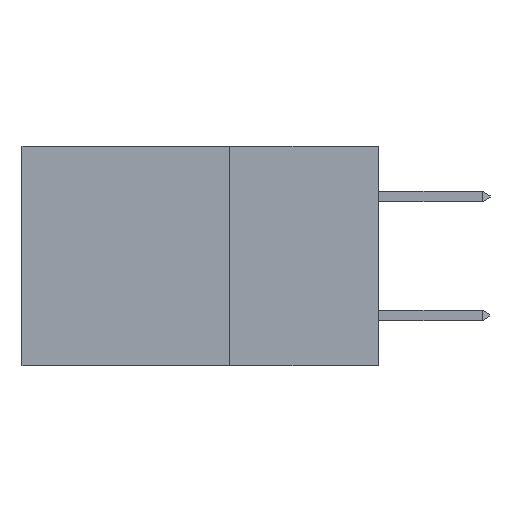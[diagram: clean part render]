
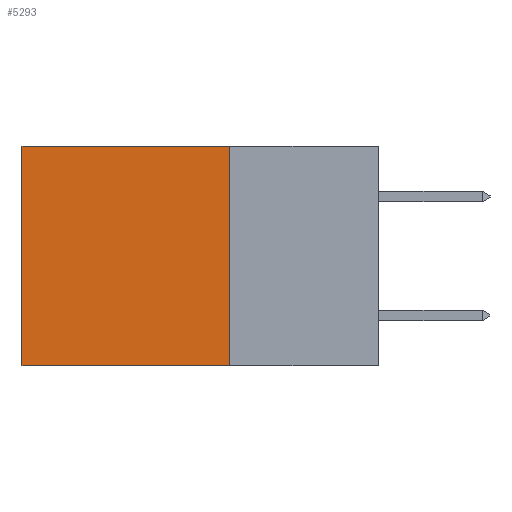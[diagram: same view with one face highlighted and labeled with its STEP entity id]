
A CAD part, left-side view. The second image highlights one B-rep face of the part: STEP entity #5293.
In plain terms, the highlighted planar face has unit normal (-1, 0, 0).
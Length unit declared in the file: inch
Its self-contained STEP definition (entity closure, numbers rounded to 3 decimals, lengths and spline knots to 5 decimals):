
#200 = VERTEX_POINT ( 'NONE', #7161 ) ;
#597 = LINE ( 'NONE', #3033, #8702 ) ;
#736 = EDGE_CURVE ( 'NONE', #4060, #6956, #4952, .T. ) ;
#774 = EDGE_CURVE ( 'NONE', #200, #6956, #8485, .T. ) ;
#1307 = EDGE_LOOP ( 'NONE', ( #2714, #2326, #4616, #5127 ) ) ;
#1610 = EDGE_CURVE ( 'NONE', #3892, #4060, #4056, .T. ) ;
#2326 = ORIENTED_EDGE ( 'NONE', *, *, #736, .F. ) ;
#2632 = CARTESIAN_POINT ( 'NONE',  ( 0.298, 0.6, -0.37 ) ) ;
#2685 = DIRECTION ( 'NONE',  ( 0., 0., -1. ) ) ;
#2714 = ORIENTED_EDGE ( 'NONE', *, *, #774, .T. ) ;
#3033 = CARTESIAN_POINT ( 'NONE',  ( 0.298, 0.25, 0. ) ) ;
#3379 = CARTESIAN_POINT ( 'NONE',  ( 0.298, 0.25, -0.37 ) ) ;
#3395 = DIRECTION ( 'NONE',  ( 1., 0., 0. ) ) ;
#3562 = DIRECTION ( 'NONE',  ( 0., 1., 0. ) ) ;
#3892 = VERTEX_POINT ( 'NONE', #9417 ) ;
#4056 = LINE ( 'NONE', #4719, #7890 ) ;
#4060 = VERTEX_POINT ( 'NONE', #8910 ) ;
#4616 = ORIENTED_EDGE ( 'NONE', *, *, #1610, .F. ) ;
#4693 = VECTOR ( 'NONE', #9692, 39.37008 ) ;
#4719 = CARTESIAN_POINT ( 'NONE',  ( 0.298, 0.25, 0. ) ) ;
#4800 = DIRECTION ( 'NONE',  ( 0., 0., -1. ) ) ;
#4940 = FACE_OUTER_BOUND ( 'NONE', #1307, .T. ) ;
#4952 = LINE ( 'NONE', #3379, #4693 ) ;
#5127 = ORIENTED_EDGE ( 'NONE', *, *, #5298, .T. ) ;
#5293 = ADVANCED_FACE ( 'NONE', ( #4940 ), #7371, .F. ) ;
#5298 = EDGE_CURVE ( 'NONE', #3892, #200, #597, .T. ) ;
#6887 = AXIS2_PLACEMENT_3D ( 'NONE', #7405, #3395, #2685 ) ;
#6956 = VERTEX_POINT ( 'NONE', #2632 ) ;
#7161 = CARTESIAN_POINT ( 'NONE',  ( 0.298, 0.6, 0. ) ) ;
#7371 = PLANE ( 'NONE',  #6887 ) ;
#7405 = CARTESIAN_POINT ( 'NONE',  ( 0.298, 0.25, 0. ) ) ;
#7890 = VECTOR ( 'NONE', #4800, 39.37008 ) ;
#8251 = VECTOR ( 'NONE', #8418, 39.37008 ) ;
#8295 = CARTESIAN_POINT ( 'NONE',  ( 0.298, 0.6, 0. ) ) ;
#8418 = DIRECTION ( 'NONE',  ( 0., 0., -1. ) ) ;
#8485 = LINE ( 'NONE', #8295, #8251 ) ;
#8702 = VECTOR ( 'NONE', #3562, 39.37008 ) ;
#8910 = CARTESIAN_POINT ( 'NONE',  ( 0.298, 0.25, -0.37 ) ) ;
#9417 = CARTESIAN_POINT ( 'NONE',  ( 0.298, 0.25, 0. ) ) ;
#9692 = DIRECTION ( 'NONE',  ( 0., 1., 0. ) ) ;
